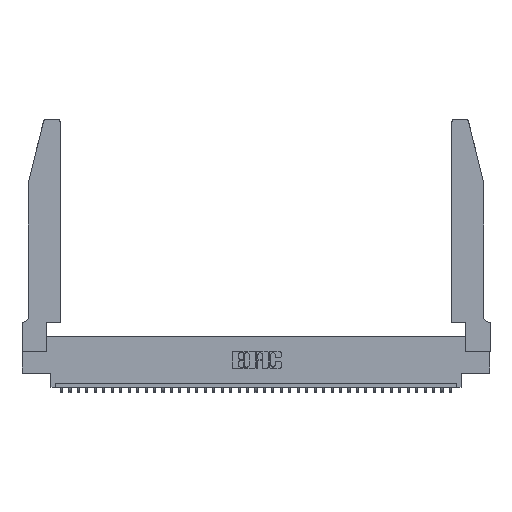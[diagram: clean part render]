
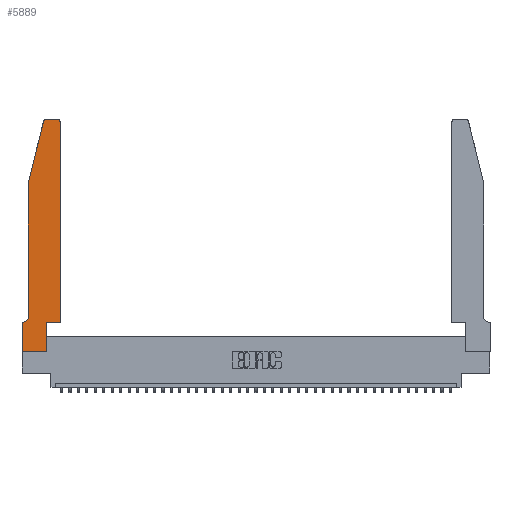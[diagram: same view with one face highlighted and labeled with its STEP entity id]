
A CAD part, top view. The second image highlights one B-rep face of the part: STEP entity #5889.
In plain terms, the highlighted planar face has unit normal (0, 0, 1).
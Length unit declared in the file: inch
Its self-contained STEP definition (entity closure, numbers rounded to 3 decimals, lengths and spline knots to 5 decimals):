
#173 = VERTEX_POINT ( 'NONE', #3155 ) ;
#430 = ORIENTED_EDGE ( 'NONE', *, *, #17171, .T. ) ;
#1925 = ORIENTED_EDGE ( 'NONE', *, *, #6057, .T. ) ;
#3155 = CARTESIAN_POINT ( 'NONE',  ( 0., 0.35, 0.37 ) ) ;
#4119 = VERTEX_POINT ( 'NONE', #10679 ) ;
#5310 = DIRECTION ( 'NONE',  ( 1., 0., 0. ) ) ;
#5889 = ADVANCED_FACE ( 'NONE', ( #18071 ), #10919, .T. ) ;
#5972 = CARTESIAN_POINT ( 'NONE',  ( 0., 0., 0.37 ) ) ;
#6057 = EDGE_CURVE ( 'NONE', #29804, #27754, #15580, .T. ) ;
#7196 = DIRECTION ( 'NONE',  ( 0., 0., -1. ) ) ;
#7537 = EDGE_CURVE ( 'NONE', #23699, #34769, #9650, .T. ) ;
#7742 = ORIENTED_EDGE ( 'NONE', *, *, #31285, .T. ) ;
#7789 = CARTESIAN_POINT ( 'NONE',  ( 0.4505, 0.35, 0.37 ) ) ;
#7842 = ORIENTED_EDGE ( 'NONE', *, *, #32630, .T. ) ;
#7956 = EDGE_CURVE ( 'NONE', #20948, #18826, #13491, .T. ) ;
#8063 = DIRECTION ( 'NONE',  ( 1., 0., 0. ) ) ;
#8146 = VERTEX_POINT ( 'NONE', #12535 ) ;
#8581 = CARTESIAN_POINT ( 'NONE',  ( 0.2865, 0.35, 0.37 ) ) ;
#8857 = DIRECTION ( 'NONE',  ( 0., 0., 1. ) ) ;
#9111 = VERTEX_POINT ( 'NONE', #26179 ) ;
#9650 = LINE ( 'NONE', #7789, #39471 ) ;
#9666 = DIRECTION ( 'NONE',  ( 0., 1., 0. ) ) ;
#9988 = DIRECTION ( 'NONE',  ( 0., -1., 0. ) ) ;
#10406 = CARTESIAN_POINT ( 'NONE',  ( 0., 0., 0.37 ) ) ;
#10679 = CARTESIAN_POINT ( 'NONE',  ( 0.4205, 2.75, 0.37 ) ) ;
#10919 = PLANE ( 'NONE',  #18100 ) ;
#11338 = ORIENTED_EDGE ( 'NONE', *, *, #34431, .T. ) ;
#11819 = CARTESIAN_POINT ( 'NONE',  ( 0.284, 2.72, 0.37 ) ) ;
#11831 = ORIENTED_EDGE ( 'NONE', *, *, #39499, .T. ) ;
#12145 = EDGE_CURVE ( 'NONE', #34769, #4119, #23274, .T. ) ;
#12525 = EDGE_CURVE ( 'NONE', #18826, #9111, #14537, .T. ) ;
#12535 = CARTESIAN_POINT ( 'NONE',  ( 0.284, 2.75, 0.37 ) ) ;
#13173 = LINE ( 'NONE', #10406, #28161 ) ;
#13328 = DIRECTION ( 'NONE',  ( -1., 0., 0. ) ) ;
#13478 = DIRECTION ( 'NONE',  ( 0., 0., 1. ) ) ;
#13484 = CARTESIAN_POINT ( 'NONE',  ( 0.2865, 0., 0.37 ) ) ;
#13491 = LINE ( 'NONE', #30496, #38972 ) ;
#13654 = VECTOR ( 'NONE', #20989, 39.37008 ) ;
#14537 = LINE ( 'NONE', #28659, #16463 ) ;
#14657 = CARTESIAN_POINT ( 'NONE',  ( 0., 0.35, 0.37 ) ) ;
#15455 = VERTEX_POINT ( 'NONE', #33219 ) ;
#15580 = LINE ( 'NONE', #8581, #13654 ) ;
#15966 = DIRECTION ( 'NONE',  ( -1., 0., 0. ) ) ;
#16463 = VECTOR ( 'NONE', #19766, 39.37008 ) ;
#16728 = DIRECTION ( 'NONE',  ( 1., 0., 0. ) ) ;
#17171 = EDGE_CURVE ( 'NONE', #8146, #20948, #24363, .T. ) ;
#17329 = AXIS2_PLACEMENT_3D ( 'NONE', #32219, #7196, #13328 ) ;
#17549 = AXIS2_PLACEMENT_3D ( 'NONE', #32107, #13478, #16728 ) ;
#18071 = FACE_OUTER_BOUND ( 'NONE', #36311, .T. ) ;
#18100 = AXIS2_PLACEMENT_3D ( 'NONE', #14657, #38542, #36212 ) ;
#18826 = VERTEX_POINT ( 'NONE', #33367 ) ;
#18983 = ORIENTED_EDGE ( 'NONE', *, *, #12145, .T. ) ;
#19490 = CARTESIAN_POINT ( 'NONE',  ( 0.0055, 0.35, 0.37 ) ) ;
#19766 = DIRECTION ( 'NONE',  ( 0., -1., 0. ) ) ;
#20948 = VERTEX_POINT ( 'NONE', #34946 ) ;
#20989 = DIRECTION ( 'NONE',  ( 0., 1., 0. ) ) ;
#21060 = CARTESIAN_POINT ( 'NONE',  ( 0.2605, 2.75, 0.37 ) ) ;
#21841 = CARTESIAN_POINT ( 'NONE',  ( 0.4505, 2.72, 0.37 ) ) ;
#22805 = CIRCLE ( 'NONE', #17329, 0.07 ) ;
#23274 = CIRCLE ( 'NONE', #17549, 0.03 ) ;
#23699 = VERTEX_POINT ( 'NONE', #26402 ) ;
#24023 = ORIENTED_EDGE ( 'NONE', *, *, #7537, .T. ) ;
#24109 = VERTEX_POINT ( 'NONE', #19490 ) ;
#24316 = EDGE_CURVE ( 'NONE', #173, #15455, #13173, .T. ) ;
#24363 = CIRCLE ( 'NONE', #24818, 0.03 ) ;
#24818 = AXIS2_PLACEMENT_3D ( 'NONE', #11819, #8857, #5310 ) ;
#25582 = LINE ( 'NONE', #32090, #35166 ) ;
#25611 = VECTOR ( 'NONE', #15966, 39.37008 ) ;
#26179 = CARTESIAN_POINT ( 'NONE',  ( 0.0755, 0.42, 0.37 ) ) ;
#26198 = EDGE_CURVE ( 'NONE', #24109, #173, #25582, .T. ) ;
#26402 = CARTESIAN_POINT ( 'NONE',  ( 0.4505, 0.35, 0.37 ) ) ;
#26472 = CARTESIAN_POINT ( 'NONE',  ( 0.4505, 0.35, 0.37 ) ) ;
#26679 = CARTESIAN_POINT ( 'NONE',  ( 0.2865, 0.35, 0.37 ) ) ;
#27468 = DIRECTION ( 'NONE',  ( 1., 0., 0. ) ) ;
#27754 = VERTEX_POINT ( 'NONE', #26679 ) ;
#27861 = LINE ( 'NONE', #26472, #33160 ) ;
#27976 = VECTOR ( 'NONE', #27468, 39.37008 ) ;
#28161 = VECTOR ( 'NONE', #9988, 39.37008 ) ;
#28659 = CARTESIAN_POINT ( 'NONE',  ( 0.0755, 2., 0.37 ) ) ;
#28961 = ORIENTED_EDGE ( 'NONE', *, *, #24316, .T. ) ;
#29804 = VERTEX_POINT ( 'NONE', #13484 ) ;
#30293 = ORIENTED_EDGE ( 'NONE', *, *, #26198, .T. ) ;
#30496 = CARTESIAN_POINT ( 'NONE',  ( 0.0755, 2., 0.37 ) ) ;
#31285 = EDGE_CURVE ( 'NONE', #9111, #24109, #22805, .T. ) ;
#32090 = CARTESIAN_POINT ( 'NONE',  ( 0.0755, 0.35, 0.37 ) ) ;
#32107 = CARTESIAN_POINT ( 'NONE',  ( 0.4205, 2.72, 0.37 ) ) ;
#32219 = CARTESIAN_POINT ( 'NONE',  ( 0.0055, 0.42, 0.37 ) ) ;
#32496 = DIRECTION ( 'NONE',  ( -1., 0., 0. ) ) ;
#32630 = EDGE_CURVE ( 'NONE', #4119, #8146, #33769, .T. ) ;
#33160 = VECTOR ( 'NONE', #8063, 39.37008 ) ;
#33219 = CARTESIAN_POINT ( 'NONE',  ( 0., 0., 0.37 ) ) ;
#33367 = CARTESIAN_POINT ( 'NONE',  ( 0.0755, 2., 0.37 ) ) ;
#33769 = LINE ( 'NONE', #21060, #25611 ) ;
#34431 = EDGE_CURVE ( 'NONE', #27754, #23699, #27861, .T. ) ;
#34769 = VERTEX_POINT ( 'NONE', #21841 ) ;
#34946 = CARTESIAN_POINT ( 'NONE',  ( 0.25487, 2.72718, 0.37 ) ) ;
#35166 = VECTOR ( 'NONE', #32496, 39.37008 ) ;
#36158 = ORIENTED_EDGE ( 'NONE', *, *, #12525, .T. ) ;
#36180 = LINE ( 'NONE', #5972, #27976 ) ;
#36212 = DIRECTION ( 'NONE',  ( 1., 0., 0. ) ) ;
#36311 = EDGE_LOOP ( 'NONE', ( #7842, #430, #37846, #36158, #7742, #30293, #28961, #11831, #1925, #11338, #24023, #18983 ) ) ;
#36542 = DIRECTION ( 'NONE',  ( -0.239, -0.971, 0. ) ) ;
#37846 = ORIENTED_EDGE ( 'NONE', *, *, #7956, .T. ) ;
#38542 = DIRECTION ( 'NONE',  ( 0., 0., 1. ) ) ;
#38972 = VECTOR ( 'NONE', #36542, 39.37008 ) ;
#39471 = VECTOR ( 'NONE', #9666, 39.37008 ) ;
#39499 = EDGE_CURVE ( 'NONE', #15455, #29804, #36180, .T. ) ;
